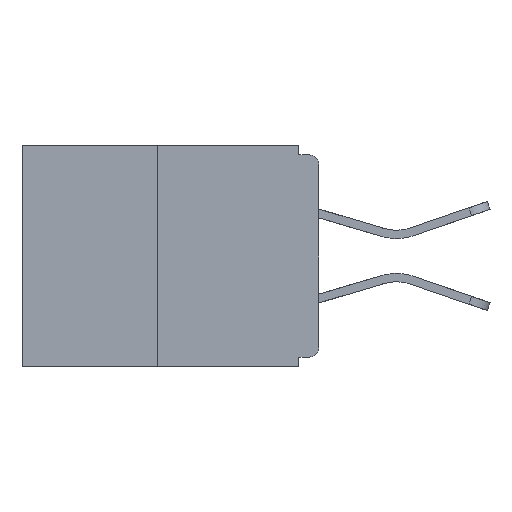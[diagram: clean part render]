
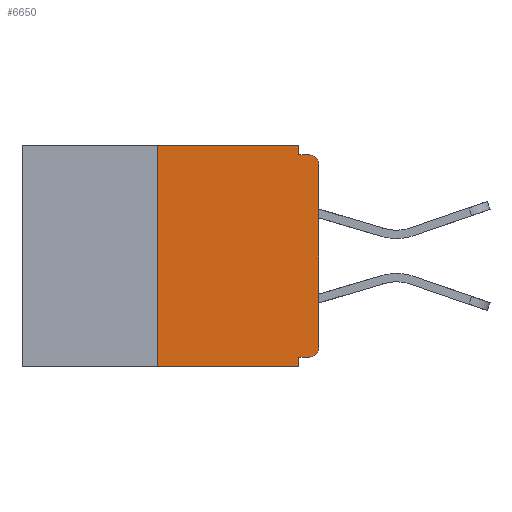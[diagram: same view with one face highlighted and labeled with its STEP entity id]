
A CAD part, left-side view. The second image highlights one B-rep face of the part: STEP entity #6650.
In plain terms, the highlighted planar face has unit normal (-1, 0, 0).
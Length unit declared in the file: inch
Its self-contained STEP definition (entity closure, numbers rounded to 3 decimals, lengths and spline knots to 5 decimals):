
#206 = VERTEX_POINT ( 'NONE', #12062 ) ;
#292 = DIRECTION ( 'NONE',  ( 0., 0., -1. ) ) ;
#401 = ORIENTED_EDGE ( 'NONE', *, *, #10813, .T. ) ;
#539 = VERTEX_POINT ( 'NONE', #19718 ) ;
#719 = DIRECTION ( 'NONE',  ( 0., 0., 1. ) ) ;
#1021 = LINE ( 'NONE', #13924, #12131 ) ;
#1088 = ORIENTED_EDGE ( 'NONE', *, *, #11150, .T. ) ;
#1094 = VERTEX_POINT ( 'NONE', #13182 ) ;
#1367 = EDGE_CURVE ( 'NONE', #206, #18345, #17697, .T. ) ;
#1370 = VECTOR ( 'NONE', #16040, 39.37008 ) ;
#1387 = VECTOR ( 'NONE', #7277, 39.37008 ) ;
#1829 = ORIENTED_EDGE ( 'NONE', *, *, #12497, .F. ) ;
#1895 = CARTESIAN_POINT ( 'NONE',  ( 0., 0.015, -0.313 ) ) ;
#2055 = CARTESIAN_POINT ( 'NONE',  ( 0., 0.46, 0. ) ) ;
#2902 = EDGE_CURVE ( 'NONE', #14988, #7312, #17418, .T. ) ;
#3511 = CARTESIAN_POINT ( 'NONE',  ( 0., 0.031, -0.328 ) ) ;
#3559 = LINE ( 'NONE', #11805, #13825 ) ;
#3635 = EDGE_CURVE ( 'NONE', #16113, #21193, #10155, .T. ) ;
#3927 = DIRECTION ( 'NONE',  ( 0., 0., 1. ) ) ;
#4363 = EDGE_LOOP ( 'NONE', ( #6029, #16489, #9289, #1829, #4841, #401, #16772, #1088, #17607, #21190 ) ) ;
#4706 = CARTESIAN_POINT ( 'NONE',  ( 0., 0.25, -0.343 ) ) ;
#4762 = CARTESIAN_POINT ( 'NONE',  ( 0., 0., -0.03 ) ) ;
#4841 = ORIENTED_EDGE ( 'NONE', *, *, #3635, .F. ) ;
#5081 = EDGE_CURVE ( 'NONE', #539, #19072, #1021, .T. ) ;
#5342 = VECTOR ( 'NONE', #719, 39.37008 ) ;
#6029 = ORIENTED_EDGE ( 'NONE', *, *, #20053, .F. ) ;
#6527 = DIRECTION ( 'NONE',  ( 0., -1., 0. ) ) ;
#6650 = ADVANCED_FACE ( 'NONE', ( #16743 ), #15135, .F. ) ;
#6670 = VECTOR ( 'NONE', #6527, 39.37008 ) ;
#6886 = AXIS2_PLACEMENT_3D ( 'NONE', #2055, #8525, #292 ) ;
#7277 = DIRECTION ( 'NONE',  ( 0., 0., -1. ) ) ;
#7312 = VERTEX_POINT ( 'NONE', #9890 ) ;
#7737 = CARTESIAN_POINT ( 'NONE',  ( 0., 0.015, -0.03 ) ) ;
#8513 = DIRECTION ( 'NONE',  ( 0., 0., -1. ) ) ;
#8525 = DIRECTION ( 'NONE',  ( 1., 0., 0. ) ) ;
#8832 = DIRECTION ( 'NONE',  ( 0., -1., 0. ) ) ;
#9232 = LINE ( 'NONE', #19668, #6670 ) ;
#9287 = VECTOR ( 'NONE', #9972, 39.37008 ) ;
#9289 = ORIENTED_EDGE ( 'NONE', *, *, #16247, .T. ) ;
#9890 = CARTESIAN_POINT ( 'NONE',  ( 0., 0.25, 0. ) ) ;
#9972 = DIRECTION ( 'NONE',  ( 0., -1., 0. ) ) ;
#10155 = LINE ( 'NONE', #20983, #1370 ) ;
#10694 = LINE ( 'NONE', #17216, #1387 ) ;
#10813 = EDGE_CURVE ( 'NONE', #16113, #206, #19018, .T. ) ;
#11037 = DIRECTION ( 'NONE',  ( -1., 0., 0. ) ) ;
#11150 = EDGE_CURVE ( 'NONE', #18345, #19072, #12079, .T. ) ;
#11585 = CARTESIAN_POINT ( 'NONE',  ( 0., 0.25, 0. ) ) ;
#11805 = CARTESIAN_POINT ( 'NONE',  ( 0., 0.031, -0.343 ) ) ;
#11811 = DIRECTION ( 'NONE',  ( 0., 0., -1. ) ) ;
#11884 = LINE ( 'NONE', #14792, #9287 ) ;
#12062 = CARTESIAN_POINT ( 'NONE',  ( 0., 0., -0.313 ) ) ;
#12079 = CIRCLE ( 'NONE', #13473, 0.015 ) ;
#12131 = VECTOR ( 'NONE', #8832, 39.37008 ) ;
#12497 = EDGE_CURVE ( 'NONE', #21193, #15670, #3559, .T. ) ;
#12704 = DIRECTION ( 'NONE',  ( 0., 0., -1. ) ) ;
#13182 = CARTESIAN_POINT ( 'NONE',  ( 0., 0.031, 0. ) ) ;
#13414 = DIRECTION ( 'NONE',  ( -1., 0., 0. ) ) ;
#13425 = EDGE_CURVE ( 'NONE', #1094, #539, #10694, .T. ) ;
#13464 = CARTESIAN_POINT ( 'NONE',  ( 0., 0.015, -0.328 ) ) ;
#13473 = AXIS2_PLACEMENT_3D ( 'NONE', #7737, #11037, #12704 ) ;
#13825 = VECTOR ( 'NONE', #8513, 39.37008 ) ;
#13924 = CARTESIAN_POINT ( 'NONE',  ( 0., 0., -0.015 ) ) ;
#14792 = CARTESIAN_POINT ( 'NONE',  ( 0., 0.46, 0. ) ) ;
#14988 = VERTEX_POINT ( 'NONE', #4706 ) ;
#15135 = PLANE ( 'NONE',  #6886 ) ;
#15670 = VERTEX_POINT ( 'NONE', #16676 ) ;
#16040 = DIRECTION ( 'NONE',  ( 0., 1., 0. ) ) ;
#16113 = VERTEX_POINT ( 'NONE', #13464 ) ;
#16247 = EDGE_CURVE ( 'NONE', #14988, #15670, #9232, .T. ) ;
#16359 = AXIS2_PLACEMENT_3D ( 'NONE', #1895, #13414, #11811 ) ;
#16489 = ORIENTED_EDGE ( 'NONE', *, *, #2902, .F. ) ;
#16676 = CARTESIAN_POINT ( 'NONE',  ( 0., 0.031, -0.343 ) ) ;
#16743 = FACE_OUTER_BOUND ( 'NONE', #4363, .T. ) ;
#16772 = ORIENTED_EDGE ( 'NONE', *, *, #1367, .T. ) ;
#17201 = VECTOR ( 'NONE', #3927, 39.37008 ) ;
#17216 = CARTESIAN_POINT ( 'NONE',  ( 0., 0.031, 0. ) ) ;
#17418 = LINE ( 'NONE', #11585, #5342 ) ;
#17607 = ORIENTED_EDGE ( 'NONE', *, *, #5081, .F. ) ;
#17697 = LINE ( 'NONE', #17916, #17201 ) ;
#17916 = CARTESIAN_POINT ( 'NONE',  ( 0., 0., 0. ) ) ;
#18345 = VERTEX_POINT ( 'NONE', #4762 ) ;
#19018 = CIRCLE ( 'NONE', #16359, 0.015 ) ;
#19072 = VERTEX_POINT ( 'NONE', #19948 ) ;
#19668 = CARTESIAN_POINT ( 'NONE',  ( 0., 0.46, -0.343 ) ) ;
#19718 = CARTESIAN_POINT ( 'NONE',  ( 0., 0.031, -0.015 ) ) ;
#19948 = CARTESIAN_POINT ( 'NONE',  ( 0., 0.015, -0.015 ) ) ;
#20053 = EDGE_CURVE ( 'NONE', #7312, #1094, #11884, .T. ) ;
#20983 = CARTESIAN_POINT ( 'NONE',  ( 0., 0., -0.328 ) ) ;
#21190 = ORIENTED_EDGE ( 'NONE', *, *, #13425, .F. ) ;
#21193 = VERTEX_POINT ( 'NONE', #3511 ) ;
